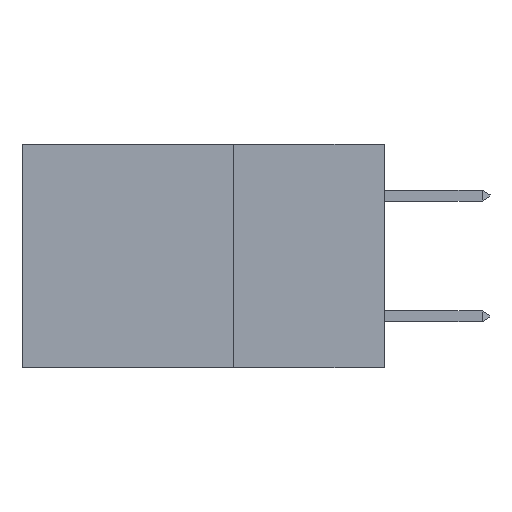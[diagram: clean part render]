
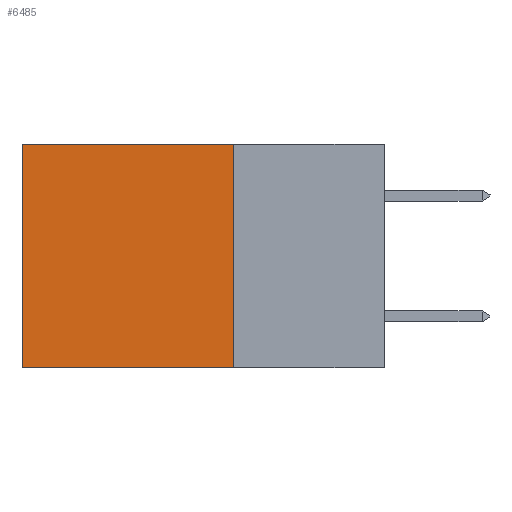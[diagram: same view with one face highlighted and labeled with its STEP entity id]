
A CAD part, left-side view. The second image highlights one B-rep face of the part: STEP entity #6485.
In plain terms, the highlighted planar face has unit normal (-1, 0, 0).
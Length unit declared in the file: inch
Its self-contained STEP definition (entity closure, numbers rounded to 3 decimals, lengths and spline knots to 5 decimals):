
#510 = FACE_OUTER_BOUND ( 'NONE', #20290, .T. ) ;
#1080 = DIRECTION ( 'NONE',  ( 0., 1., 0. ) ) ;
#4115 = DIRECTION ( 'NONE',  ( 0., 0., -1. ) ) ;
#6485 = ADVANCED_FACE ( 'NONE', ( #510 ), #15907, .F. ) ;
#8166 = ORIENTED_EDGE ( 'NONE', *, *, #41345, .T. ) ;
#8344 = CARTESIAN_POINT ( 'NONE',  ( 0.2875, 0.6, 0. ) ) ;
#10567 = LINE ( 'NONE', #17990, #27252 ) ;
#10747 = DIRECTION ( 'NONE',  ( 0., 0., -1. ) ) ;
#10981 = EDGE_CURVE ( 'NONE', #34306, #15571, #24167, .T. ) ;
#11388 = EDGE_CURVE ( 'NONE', #33402, #15571, #10567, .T. ) ;
#12209 = VECTOR ( 'NONE', #4115, 39.37008 ) ;
#14378 = CARTESIAN_POINT ( 'NONE',  ( 0.2875, 0.25, 0. ) ) ;
#15571 = VERTEX_POINT ( 'NONE', #16651 ) ;
#15618 = CARTESIAN_POINT ( 'NONE',  ( 0.2875, 0.25, 0. ) ) ;
#15907 = PLANE ( 'NONE',  #39771 ) ;
#16651 = CARTESIAN_POINT ( 'NONE',  ( 0.2875, 0.6, -0.37 ) ) ;
#16888 = LINE ( 'NONE', #14378, #12209 ) ;
#17338 = CARTESIAN_POINT ( 'NONE',  ( 0.2875, 0.25, 0. ) ) ;
#17820 = CARTESIAN_POINT ( 'NONE',  ( 0.2875, 0.6, 0. ) ) ;
#17861 = ORIENTED_EDGE ( 'NONE', *, *, #43269, .F. ) ;
#17990 = CARTESIAN_POINT ( 'NONE',  ( 0.2875, 0.25, -0.37 ) ) ;
#18834 = DIRECTION ( 'NONE',  ( 1., 0., 0. ) ) ;
#20290 = EDGE_LOOP ( 'NONE', ( #36053, #36049, #17861, #8166 ) ) ;
#22299 = DIRECTION ( 'NONE',  ( 0., 1., 0. ) ) ;
#22481 = LINE ( 'NONE', #24185, #39786 ) ;
#24167 = LINE ( 'NONE', #8344, #30954 ) ;
#24185 = CARTESIAN_POINT ( 'NONE',  ( 0.2875, 0.25, 0. ) ) ;
#27252 = VECTOR ( 'NONE', #22299, 39.37008 ) ;
#30954 = VECTOR ( 'NONE', #10747, 39.37008 ) ;
#32478 = CARTESIAN_POINT ( 'NONE',  ( 0.2875, 0.25, -0.37 ) ) ;
#33402 = VERTEX_POINT ( 'NONE', #32478 ) ;
#34306 = VERTEX_POINT ( 'NONE', #17820 ) ;
#35865 = DIRECTION ( 'NONE',  ( 0., 0., -1. ) ) ;
#36049 = ORIENTED_EDGE ( 'NONE', *, *, #11388, .F. ) ;
#36053 = ORIENTED_EDGE ( 'NONE', *, *, #10981, .T. ) ;
#37361 = VERTEX_POINT ( 'NONE', #17338 ) ;
#39771 = AXIS2_PLACEMENT_3D ( 'NONE', #15618, #18834, #35865 ) ;
#39786 = VECTOR ( 'NONE', #1080, 39.37008 ) ;
#41345 = EDGE_CURVE ( 'NONE', #37361, #34306, #22481, .T. ) ;
#43269 = EDGE_CURVE ( 'NONE', #37361, #33402, #16888, .T. ) ;
